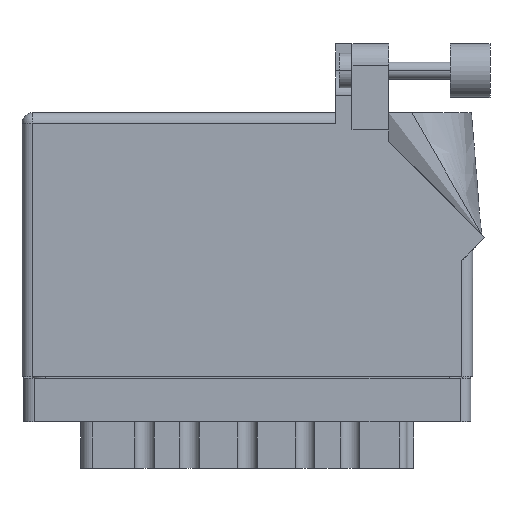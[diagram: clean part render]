
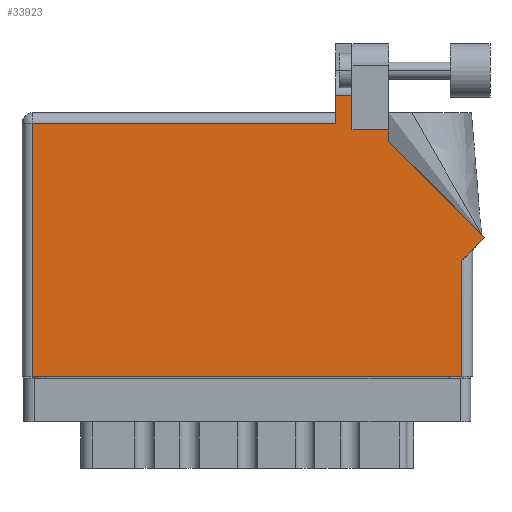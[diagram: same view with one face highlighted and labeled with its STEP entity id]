
A CAD part, front view. The second image highlights one B-rep face of the part: STEP entity #33923.
In plain terms, the highlighted face is planar.
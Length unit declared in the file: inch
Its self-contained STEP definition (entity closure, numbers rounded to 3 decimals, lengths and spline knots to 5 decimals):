
#286 = DIRECTION ( 'NONE',  ( -1., 0., 0. ) ) ;
#393 = LINE ( 'NONE', #7969, #636 ) ;
#548 = EDGE_CURVE ( 'NONE', #40459, #15834, #17741, .T. ) ;
#622 = ORIENTED_EDGE ( 'NONE', *, *, #4092, .T. ) ;
#636 = VECTOR ( 'NONE', #34475, 39.37008 ) ;
#1660 = CARTESIAN_POINT ( 'NONE',  ( 2.126, 1.43, 0. ) ) ;
#1925 = FACE_OUTER_BOUND ( 'NONE', #43348, .T. ) ;
#2466 = ORIENTED_EDGE ( 'NONE', *, *, #41002, .T. ) ;
#2837 = DIRECTION ( 'NONE',  ( 1., 0., 0. ) ) ;
#4092 = EDGE_CURVE ( 'NONE', #15834, #6082, #21257, .T. ) ;
#5690 = CARTESIAN_POINT ( 'NONE',  ( 1.913, 1.43, 0. ) ) ;
#6082 = VERTEX_POINT ( 'NONE', #28994 ) ;
#6104 = DIRECTION ( 'NONE',  ( 0., 1., 0. ) ) ;
#6516 = VERTEX_POINT ( 'NONE', #7280 ) ;
#6636 = VECTOR ( 'NONE', #37849, 39.37008 ) ;
#6880 = CARTESIAN_POINT ( 'NONE',  ( 0., 0., 0. ) ) ;
#7280 = CARTESIAN_POINT ( 'NONE',  ( 1.819, 1.6315, 0. ) ) ;
#7969 = CARTESIAN_POINT ( 'NONE',  ( 1.819, 1.53, 0. ) ) ;
#8845 = VECTOR ( 'NONE', #286, 39.37008 ) ;
#8994 = VERTEX_POINT ( 'NONE', #42185 ) ;
#9343 = LINE ( 'NONE', #34048, #26668 ) ;
#9889 = EDGE_CURVE ( 'NONE', #14551, #8994, #10976, .T. ) ;
#10976 = LINE ( 'NONE', #26357, #12239 ) ;
#10990 = CARTESIAN_POINT ( 'NONE',  ( 2.126, 1.36442, 0. ) ) ;
#11485 = LINE ( 'NONE', #31408, #48413 ) ;
#11721 = DIRECTION ( 'NONE',  ( 0., 1., 0. ) ) ;
#12239 = VECTOR ( 'NONE', #11721, 39.37008 ) ;
#12815 = PLANE ( 'NONE',  #26820 ) ;
#14059 = ORIENTED_EDGE ( 'NONE', *, *, #30413, .T. ) ;
#14551 = VERTEX_POINT ( 'NONE', #5690 ) ;
#15834 = VERTEX_POINT ( 'NONE', #20608 ) ;
#16395 = ORIENTED_EDGE ( 'NONE', *, *, #47213, .T. ) ;
#17451 = VECTOR ( 'NONE', #48019, 39.37008 ) ;
#17453 = VERTEX_POINT ( 'NONE', #24593 ) ;
#17741 = LINE ( 'NONE', #6880, #32879 ) ;
#18209 = CARTESIAN_POINT ( 'NONE',  ( 2.126, 1.36442, 0. ) ) ;
#18647 = DIRECTION ( 'NONE',  ( -1., 0., 0. ) ) ;
#18657 = CARTESIAN_POINT ( 'NONE',  ( 2.612, 0.737, 0. ) ) ;
#18786 = CARTESIAN_POINT ( 'NONE',  ( 0.062, 1.468, 0. ) ) ;
#18789 = VERTEX_POINT ( 'NONE', #39553 ) ;
#18997 = VERTEX_POINT ( 'NONE', #18786 ) ;
#19668 = ORIENTED_EDGE ( 'NONE', *, *, #39654, .T. ) ;
#20608 = CARTESIAN_POINT ( 'NONE',  ( 2.55, 0., 0. ) ) ;
#21257 = LINE ( 'NONE', #44979, #27185 ) ;
#22657 = ORIENTED_EDGE ( 'NONE', *, *, #548, .T. ) ;
#23685 = VERTEX_POINT ( 'NONE', #10990 ) ;
#24593 = CARTESIAN_POINT ( 'NONE',  ( 2.68271, 0.80771, 0. ) ) ;
#26357 = CARTESIAN_POINT ( 'NONE',  ( 1.913, 1.43, 0. ) ) ;
#26668 = VECTOR ( 'NONE', #18647, 39.37008 ) ;
#26820 = AXIS2_PLACEMENT_3D ( 'NONE', #32737, #44092, #48122 ) ;
#26966 = LINE ( 'NONE', #45655, #39315 ) ;
#27135 = EDGE_CURVE ( 'NONE', #18789, #18997, #26966, .T. ) ;
#27185 = VECTOR ( 'NONE', #6104, 39.37008 ) ;
#27322 = ORIENTED_EDGE ( 'NONE', *, *, #27135, .T. ) ;
#27607 = EDGE_CURVE ( 'NONE', #6516, #18789, #393, .T. ) ;
#28994 = CARTESIAN_POINT ( 'NONE',  ( 2.55, 0.675, 0. ) ) ;
#29012 = CARTESIAN_POINT ( 'NONE',  ( 0.062, 0., 0. ) ) ;
#29638 = EDGE_CURVE ( 'NONE', #8994, #6516, #30603, .T. ) ;
#29846 = ORIENTED_EDGE ( 'NONE', *, *, #29638, .T. ) ;
#30413 = EDGE_CURVE ( 'NONE', #17453, #23685, #11485, .T. ) ;
#30603 = LINE ( 'NONE', #45983, #8845 ) ;
#31408 = CARTESIAN_POINT ( 'NONE',  ( 2.68271, 0.80771, 0. ) ) ;
#32737 = CARTESIAN_POINT ( 'NONE',  ( 0., 1.53, 0. ) ) ;
#32879 = VECTOR ( 'NONE', #2837, 39.37008 ) ;
#32887 = CARTESIAN_POINT ( 'NONE',  ( 0.062, 0., 0. ) ) ;
#33239 = ORIENTED_EDGE ( 'NONE', *, *, #33467, .T. ) ;
#33467 = EDGE_CURVE ( 'NONE', #18997, #40459, #40364, .T. ) ;
#33923 = ADVANCED_FACE ( 'NONE', ( #1925 ), #12815, .F. ) ;
#34048 = CARTESIAN_POINT ( 'NONE',  ( 2.126, 1.43, 0. ) ) ;
#34475 = DIRECTION ( 'NONE',  ( 0., -1., 0. ) ) ;
#34786 = DIRECTION ( 'NONE',  ( -1., 0., 0. ) ) ;
#35887 = ORIENTED_EDGE ( 'NONE', *, *, #27607, .T. ) ;
#37849 = DIRECTION ( 'NONE',  ( 0.707, 0.707, 0. ) ) ;
#39315 = VECTOR ( 'NONE', #34786, 39.37008 ) ;
#39553 = CARTESIAN_POINT ( 'NONE',  ( 1.819, 1.468, 0. ) ) ;
#39654 = EDGE_CURVE ( 'NONE', #41766, #14551, #9343, .T. ) ;
#40364 = LINE ( 'NONE', #29012, #41308 ) ;
#40459 = VERTEX_POINT ( 'NONE', #32887 ) ;
#40801 = ORIENTED_EDGE ( 'NONE', *, *, #9889, .T. ) ;
#40933 = LINE ( 'NONE', #18209, #17451 ) ;
#41002 = EDGE_CURVE ( 'NONE', #6082, #17453, #45666, .T. ) ;
#41308 = VECTOR ( 'NONE', #44399, 39.37008 ) ;
#41766 = VERTEX_POINT ( 'NONE', #1660 ) ;
#42185 = CARTESIAN_POINT ( 'NONE',  ( 1.913, 1.6315, 0. ) ) ;
#42759 = DIRECTION ( 'NONE',  ( -0.707, 0.707, 0. ) ) ;
#43348 = EDGE_LOOP ( 'NONE', ( #40801, #29846, #35887, #27322, #33239, #22657, #622, #2466, #14059, #16395, #19668 ) ) ;
#44092 = DIRECTION ( 'NONE',  ( 0., 0., -1. ) ) ;
#44399 = DIRECTION ( 'NONE',  ( 0., -1., 0. ) ) ;
#44979 = CARTESIAN_POINT ( 'NONE',  ( 2.55, 0.737, 0. ) ) ;
#45655 = CARTESIAN_POINT ( 'NONE',  ( 0., 1.468, 0. ) ) ;
#45666 = LINE ( 'NONE', #18657, #6636 ) ;
#45983 = CARTESIAN_POINT ( 'NONE',  ( 2.24377, 1.6315, 0. ) ) ;
#47213 = EDGE_CURVE ( 'NONE', #23685, #41766, #40933, .T. ) ;
#48019 = DIRECTION ( 'NONE',  ( 0., 1., 0. ) ) ;
#48122 = DIRECTION ( 'NONE',  ( -1., 0., 0. ) ) ;
#48413 = VECTOR ( 'NONE', #42759, 39.37008 ) ;
